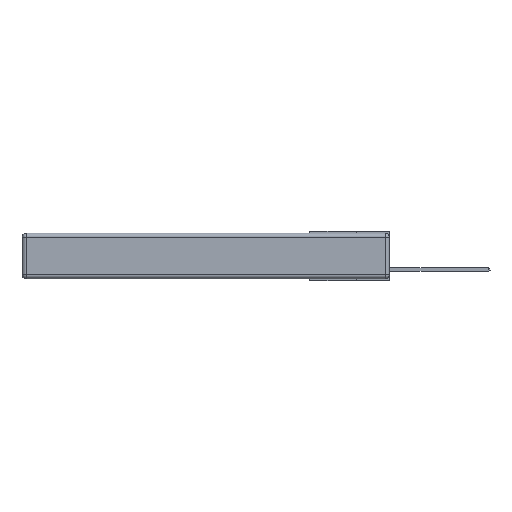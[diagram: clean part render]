
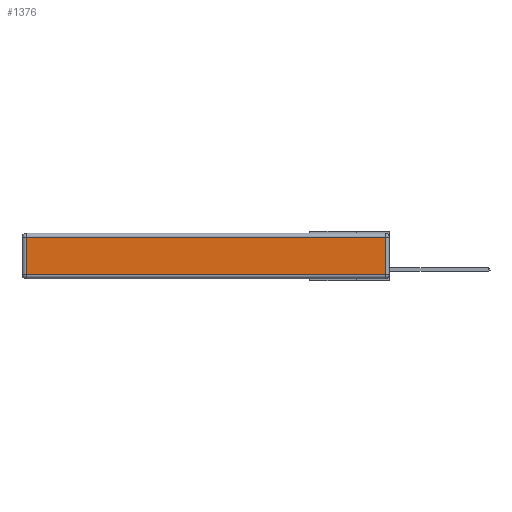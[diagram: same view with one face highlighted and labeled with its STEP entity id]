
A CAD part, left-side view. The second image highlights one B-rep face of the part: STEP entity #1376.
In plain terms, the highlighted planar face has unit normal (-1, 0, 0).
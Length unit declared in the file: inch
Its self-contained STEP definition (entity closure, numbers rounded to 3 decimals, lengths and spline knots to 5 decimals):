
#11 = EDGE_LOOP ( 'NONE', ( #6541, #13327, #8624, #9909 ) ) ;
#475 = VECTOR ( 'NONE', #6772, 39.37008 ) ;
#1376 = ADVANCED_FACE ( 'NONE', ( #9118 ), #11737, .T. ) ;
#2196 = DIRECTION ( 'NONE',  ( 0., 0., 1. ) ) ;
#2868 = LINE ( 'NONE', #8853, #14326 ) ;
#2896 = EDGE_CURVE ( 'NONE', #3305, #14965, #13967, .T. ) ;
#3305 = VERTEX_POINT ( 'NONE', #9174 ) ;
#4160 = DIRECTION ( 'NONE',  ( 0., 1., 0. ) ) ;
#4368 = VERTEX_POINT ( 'NONE', #14420 ) ;
#5549 = VECTOR ( 'NONE', #8934, 39.37008 ) ;
#6218 = EDGE_CURVE ( 'NONE', #4368, #12013, #14786, .T. ) ;
#6284 = LINE ( 'NONE', #6496, #5549 ) ;
#6496 = CARTESIAN_POINT ( 'NONE',  ( 0., 0., -0.313 ) ) ;
#6541 = ORIENTED_EDGE ( 'NONE', *, *, #12860, .T. ) ;
#6772 = DIRECTION ( 'NONE',  ( 0., 0., -1. ) ) ;
#8624 = ORIENTED_EDGE ( 'NONE', *, *, #13852, .T. ) ;
#8853 = CARTESIAN_POINT ( 'NONE',  ( 0., 2.75, -0.03 ) ) ;
#8934 = DIRECTION ( 'NONE',  ( 0., -1., 0. ) ) ;
#9118 = FACE_OUTER_BOUND ( 'NONE', #11, .T. ) ;
#9174 = CARTESIAN_POINT ( 'NONE',  ( 0., 0.03, -0.313 ) ) ;
#9410 = DIRECTION ( 'NONE',  ( -1., 0., 0. ) ) ;
#9629 = VECTOR ( 'NONE', #13445, 39.37008 ) ;
#9909 = ORIENTED_EDGE ( 'NONE', *, *, #6218, .T. ) ;
#11015 = CARTESIAN_POINT ( 'NONE',  ( 0., 2.72, -0.313 ) ) ;
#11141 = AXIS2_PLACEMENT_3D ( 'NONE', #12979, #9410, #2196 ) ;
#11737 = PLANE ( 'NONE',  #11141 ) ;
#12013 = VERTEX_POINT ( 'NONE', #11015 ) ;
#12860 = EDGE_CURVE ( 'NONE', #12013, #3305, #6284, .T. ) ;
#12979 = CARTESIAN_POINT ( 'NONE',  ( 0., 0., -0.343 ) ) ;
#13327 = ORIENTED_EDGE ( 'NONE', *, *, #2896, .T. ) ;
#13445 = DIRECTION ( 'NONE',  ( 0., 0., 1. ) ) ;
#13603 = CARTESIAN_POINT ( 'NONE',  ( 0., 0.03, -0.343 ) ) ;
#13852 = EDGE_CURVE ( 'NONE', #14965, #4368, #2868, .T. ) ;
#13949 = CARTESIAN_POINT ( 'NONE',  ( 0., 2.72, -0.343 ) ) ;
#13967 = LINE ( 'NONE', #13603, #9629 ) ;
#14273 = CARTESIAN_POINT ( 'NONE',  ( 0., 0.03, -0.03 ) ) ;
#14326 = VECTOR ( 'NONE', #4160, 39.37008 ) ;
#14420 = CARTESIAN_POINT ( 'NONE',  ( 0., 2.72, -0.03 ) ) ;
#14786 = LINE ( 'NONE', #13949, #475 ) ;
#14965 = VERTEX_POINT ( 'NONE', #14273 ) ;
